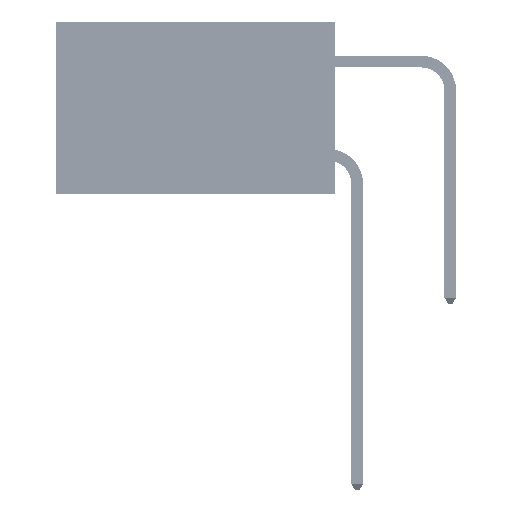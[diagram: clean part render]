
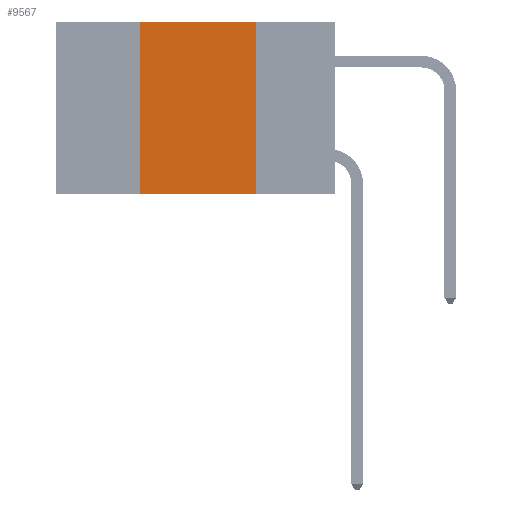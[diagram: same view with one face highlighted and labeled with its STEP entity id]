
A CAD part, left-side view. The second image highlights one B-rep face of the part: STEP entity #9567.
In plain terms, the highlighted planar face has unit normal (-1, 0, 0).
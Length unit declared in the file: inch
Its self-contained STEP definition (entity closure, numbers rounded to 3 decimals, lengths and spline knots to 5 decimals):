
#766 = DIRECTION ( 'NONE',  ( 1., 0., 0. ) ) ;
#2540 = VERTEX_POINT ( 'NONE', #35248 ) ;
#2974 = CARTESIAN_POINT ( 'NONE',  ( 0., 0.6, -0.37 ) ) ;
#4653 = LINE ( 'NONE', #38119, #19422 ) ;
#4925 = DIRECTION ( 'NONE',  ( 0., 0., 1. ) ) ;
#4973 = DIRECTION ( 'NONE',  ( 0., 0., -1. ) ) ;
#6514 = ORIENTED_EDGE ( 'NONE', *, *, #46524, .F. ) ;
#6592 = DIRECTION ( 'NONE',  ( 0., -1., 0. ) ) ;
#6755 = VECTOR ( 'NONE', #6592, 39.37008 ) ;
#8059 = ORIENTED_EDGE ( 'NONE', *, *, #13851, .T. ) ;
#8370 = EDGE_LOOP ( 'NONE', ( #23821, #6514, #45651, #8059 ) ) ;
#9567 = ADVANCED_FACE ( 'NONE', ( #34512 ), #21829, .F. ) ;
#11787 = CARTESIAN_POINT ( 'NONE',  ( 0., 0.17, -0.37 ) ) ;
#13851 = EDGE_CURVE ( 'NONE', #33859, #21925, #40344, .T. ) ;
#19422 = VECTOR ( 'NONE', #4925, 39.37008 ) ;
#20140 = VECTOR ( 'NONE', #45641, 39.37008 ) ;
#21677 = EDGE_CURVE ( 'NONE', #33859, #2540, #4653, .T. ) ;
#21829 = PLANE ( 'NONE',  #53339 ) ;
#21925 = VERTEX_POINT ( 'NONE', #11787 ) ;
#23821 = ORIENTED_EDGE ( 'NONE', *, *, #29609, .F. ) ;
#25200 = LINE ( 'NONE', #51200, #39739 ) ;
#29609 = EDGE_CURVE ( 'NONE', #40806, #21925, #25200, .T. ) ;
#33671 = CARTESIAN_POINT ( 'NONE',  ( 0., 0.6, 0. ) ) ;
#33859 = VERTEX_POINT ( 'NONE', #43560 ) ;
#34512 = FACE_OUTER_BOUND ( 'NONE', #8370, .T. ) ;
#35248 = CARTESIAN_POINT ( 'NONE',  ( 0., 0.42, 0. ) ) ;
#37975 = CARTESIAN_POINT ( 'NONE',  ( 0., 0.17, 0. ) ) ;
#38119 = CARTESIAN_POINT ( 'NONE',  ( 0., 0.42, 0. ) ) ;
#38677 = CARTESIAN_POINT ( 'NONE',  ( 0., 0.6, 0. ) ) ;
#39739 = VECTOR ( 'NONE', #4973, 39.37008 ) ;
#40344 = LINE ( 'NONE', #2974, #6755 ) ;
#40806 = VERTEX_POINT ( 'NONE', #37975 ) ;
#41198 = LINE ( 'NONE', #33671, #20140 ) ;
#43560 = CARTESIAN_POINT ( 'NONE',  ( 0., 0.42, -0.37 ) ) ;
#45641 = DIRECTION ( 'NONE',  ( 0., -1., 0. ) ) ;
#45651 = ORIENTED_EDGE ( 'NONE', *, *, #21677, .F. ) ;
#46524 = EDGE_CURVE ( 'NONE', #2540, #40806, #41198, .T. ) ;
#51200 = CARTESIAN_POINT ( 'NONE',  ( 0., 0.17, 0. ) ) ;
#51443 = DIRECTION ( 'NONE',  ( 0., 0., -1. ) ) ;
#53339 = AXIS2_PLACEMENT_3D ( 'NONE', #38677, #766, #51443 ) ;
